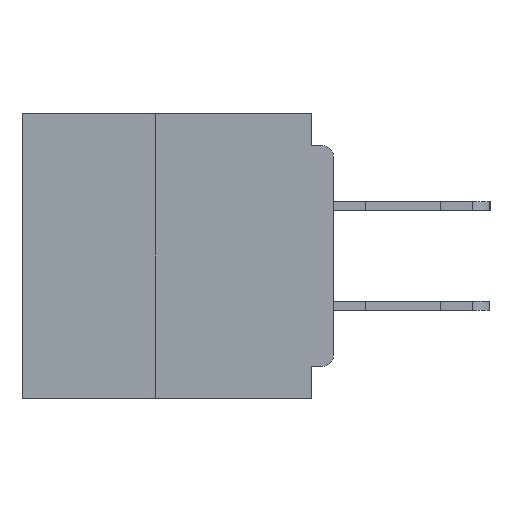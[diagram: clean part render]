
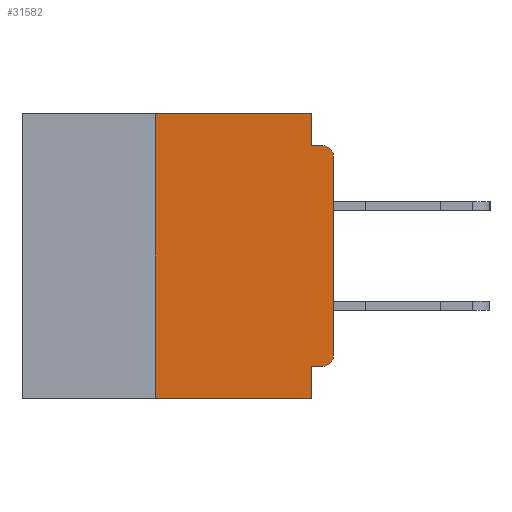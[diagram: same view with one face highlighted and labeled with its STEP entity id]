
A CAD part, left-side view. The second image highlights one B-rep face of the part: STEP entity #31582.
In plain terms, the highlighted planar face has unit normal (-1, 0, 0).
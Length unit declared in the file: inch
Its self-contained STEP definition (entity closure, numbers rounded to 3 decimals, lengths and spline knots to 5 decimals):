
#390 = CARTESIAN_POINT ( 'NONE',  ( 0., 0., -0.34 ) ) ;
#426 = VECTOR ( 'NONE', #12806, 39.37008 ) ;
#1390 = EDGE_CURVE ( 'NONE', #22096, #33675, #11608, .T. ) ;
#1573 = CARTESIAN_POINT ( 'NONE',  ( 0., 0.25, -0.4 ) ) ;
#2028 = VERTEX_POINT ( 'NONE', #8051 ) ;
#2045 = AXIS2_PLACEMENT_3D ( 'NONE', #2991, #31676, #7131 ) ;
#2991 = CARTESIAN_POINT ( 'NONE',  ( 0., 0.015, -0.34 ) ) ;
#3747 = DIRECTION ( 'NONE',  ( 0., 0., 1. ) ) ;
#5045 = PLANE ( 'NONE',  #21565 ) ;
#5331 = ORIENTED_EDGE ( 'NONE', *, *, #13011, .F. ) ;
#7131 = DIRECTION ( 'NONE',  ( 0., 0., -1. ) ) ;
#7693 = ORIENTED_EDGE ( 'NONE', *, *, #28264, .T. ) ;
#8051 = CARTESIAN_POINT ( 'NONE',  ( 0., 0.25, 0. ) ) ;
#8471 = CARTESIAN_POINT ( 'NONE',  ( 0., 0.015, -0.355 ) ) ;
#8500 = LINE ( 'NONE', #40195, #39896 ) ;
#8658 = CARTESIAN_POINT ( 'NONE',  ( 0., 0.031, -0.4 ) ) ;
#9059 = VERTEX_POINT ( 'NONE', #40366 ) ;
#9169 = CARTESIAN_POINT ( 'NONE',  ( 0., 0.437, 0. ) ) ;
#10166 = VERTEX_POINT ( 'NONE', #14440 ) ;
#10699 = ORIENTED_EDGE ( 'NONE', *, *, #48139, .F. ) ;
#11608 = LINE ( 'NONE', #12427, #21224 ) ;
#12427 = CARTESIAN_POINT ( 'NONE',  ( 0., 0., -0.045 ) ) ;
#12749 = EDGE_CURVE ( 'NONE', #41696, #10166, #34460, .T. ) ;
#12806 = DIRECTION ( 'NONE',  ( 0., 0., -1. ) ) ;
#13011 = EDGE_CURVE ( 'NONE', #2028, #9059, #50378, .T. ) ;
#13254 = ORIENTED_EDGE ( 'NONE', *, *, #41185, .F. ) ;
#13328 = DIRECTION ( 'NONE',  ( 0., 0., -1. ) ) ;
#14440 = CARTESIAN_POINT ( 'NONE',  ( 0., 0.031, -0.4 ) ) ;
#14481 = LINE ( 'NONE', #40913, #36243 ) ;
#15262 = ORIENTED_EDGE ( 'NONE', *, *, #12749, .F. ) ;
#16411 = DIRECTION ( 'NONE',  ( 0., 0., 1. ) ) ;
#17430 = VERTEX_POINT ( 'NONE', #390 ) ;
#19306 = LINE ( 'NONE', #52785, #39727 ) ;
#19848 = DIRECTION ( 'NONE',  ( 0., 1., 0. ) ) ;
#20466 = DIRECTION ( 'NONE',  ( -1., 0., 0. ) ) ;
#21118 = CARTESIAN_POINT ( 'NONE',  ( 0., 0.437, -0.4 ) ) ;
#21224 = VECTOR ( 'NONE', #32814, 39.37008 ) ;
#21565 = AXIS2_PLACEMENT_3D ( 'NONE', #9169, #37826, #13328 ) ;
#22096 = VERTEX_POINT ( 'NONE', #46239 ) ;
#22413 = EDGE_LOOP ( 'NONE', ( #7693, #34994, #51226, #13254, #5331, #45514, #40721, #15262, #10699, #30120 ) ) ;
#22472 = EDGE_CURVE ( 'NONE', #37426, #33675, #48145, .T. ) ;
#23316 = CARTESIAN_POINT ( 'NONE',  ( 0., 0.031, 0. ) ) ;
#23613 = FACE_OUTER_BOUND ( 'NONE', #22413, .T. ) ;
#25250 = DIRECTION ( 'NONE',  ( 0., -1., 0. ) ) ;
#26010 = VECTOR ( 'NONE', #25250, 39.37008 ) ;
#27387 = DIRECTION ( 'NONE',  ( 0., 0., -1. ) ) ;
#28264 = EDGE_CURVE ( 'NONE', #17430, #37426, #14481, .T. ) ;
#30120 = ORIENTED_EDGE ( 'NONE', *, *, #44405, .T. ) ;
#31582 = ADVANCED_FACE ( 'NONE', ( #23613 ), #5045, .F. ) ;
#31676 = DIRECTION ( 'NONE',  ( -1., 0., 0. ) ) ;
#31958 = AXIS2_PLACEMENT_3D ( 'NONE', #44970, #20466, #49029 ) ;
#32814 = DIRECTION ( 'NONE',  ( 0., -1., 0. ) ) ;
#33675 = VERTEX_POINT ( 'NONE', #41584 ) ;
#34460 = LINE ( 'NONE', #8658, #426 ) ;
#34730 = VECTOR ( 'NONE', #27387, 39.37008 ) ;
#34994 = ORIENTED_EDGE ( 'NONE', *, *, #22472, .T. ) ;
#36036 = LINE ( 'NONE', #23316, #34730 ) ;
#36243 = VECTOR ( 'NONE', #16411, 39.37008 ) ;
#37426 = VERTEX_POINT ( 'NONE', #47716 ) ;
#37826 = DIRECTION ( 'NONE',  ( 1., 0., 0. ) ) ;
#37889 = VERTEX_POINT ( 'NONE', #1573 ) ;
#38895 = CARTESIAN_POINT ( 'NONE',  ( 0., 0.437, 0. ) ) ;
#39076 = DIRECTION ( 'NONE',  ( 0., -1., 0. ) ) ;
#39548 = VECTOR ( 'NONE', #39076, 39.37008 ) ;
#39727 = VECTOR ( 'NONE', #3747, 39.37008 ) ;
#39896 = VECTOR ( 'NONE', #19848, 39.37008 ) ;
#40195 = CARTESIAN_POINT ( 'NONE',  ( 0., 0., -0.355 ) ) ;
#40366 = CARTESIAN_POINT ( 'NONE',  ( 0., 0.031, 0. ) ) ;
#40721 = ORIENTED_EDGE ( 'NONE', *, *, #46716, .T. ) ;
#40913 = CARTESIAN_POINT ( 'NONE',  ( 0., 0., 0. ) ) ;
#41185 = EDGE_CURVE ( 'NONE', #9059, #22096, #36036, .T. ) ;
#41584 = CARTESIAN_POINT ( 'NONE',  ( 0., 0.015, -0.045 ) ) ;
#41696 = VERTEX_POINT ( 'NONE', #46436 ) ;
#43998 = EDGE_CURVE ( 'NONE', #37889, #2028, #19306, .T. ) ;
#44405 = EDGE_CURVE ( 'NONE', #48316, #17430, #50520, .T. ) ;
#44970 = CARTESIAN_POINT ( 'NONE',  ( 0., 0.015, -0.06 ) ) ;
#45514 = ORIENTED_EDGE ( 'NONE', *, *, #43998, .F. ) ;
#46239 = CARTESIAN_POINT ( 'NONE',  ( 0., 0.031, -0.045 ) ) ;
#46436 = CARTESIAN_POINT ( 'NONE',  ( 0., 0.031, -0.355 ) ) ;
#46716 = EDGE_CURVE ( 'NONE', #37889, #10166, #47781, .T. ) ;
#47716 = CARTESIAN_POINT ( 'NONE',  ( 0., 0., -0.06 ) ) ;
#47781 = LINE ( 'NONE', #21118, #26010 ) ;
#48139 = EDGE_CURVE ( 'NONE', #48316, #41696, #8500, .T. ) ;
#48145 = CIRCLE ( 'NONE', #31958, 0.015 ) ;
#48316 = VERTEX_POINT ( 'NONE', #8471 ) ;
#49029 = DIRECTION ( 'NONE',  ( 0., 0., -1. ) ) ;
#50378 = LINE ( 'NONE', #38895, #39548 ) ;
#50520 = CIRCLE ( 'NONE', #2045, 0.015 ) ;
#51226 = ORIENTED_EDGE ( 'NONE', *, *, #1390, .F. ) ;
#52785 = CARTESIAN_POINT ( 'NONE',  ( 0., 0.25, -0.4 ) ) ;
